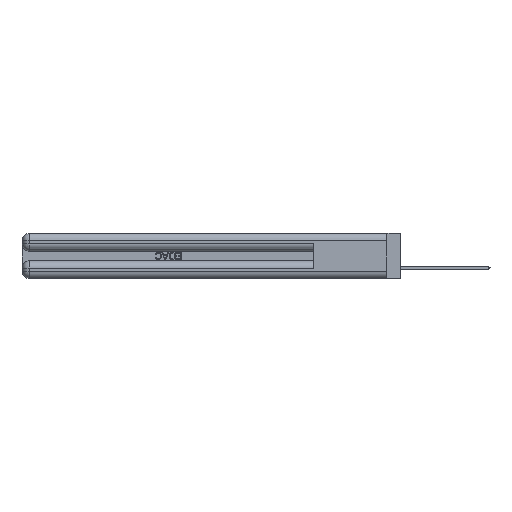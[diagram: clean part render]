
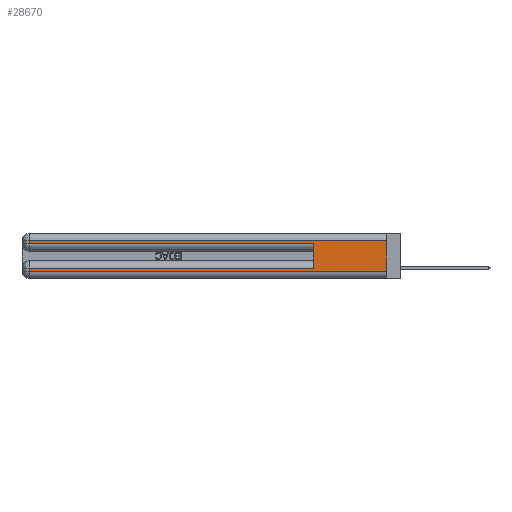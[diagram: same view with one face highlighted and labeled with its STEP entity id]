
A CAD part, left-side view. The second image highlights one B-rep face of the part: STEP entity #28670.
In plain terms, the highlighted planar face has unit normal (-1, 0, 0).
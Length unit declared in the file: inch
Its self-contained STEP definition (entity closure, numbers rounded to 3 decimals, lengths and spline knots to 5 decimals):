
#838 = LINE ( 'NONE', #39838, #31116 ) ;
#1566 = CARTESIAN_POINT ( 'NONE',  ( 0., 0., 0.06 ) ) ;
#2603 = ORIENTED_EDGE ( 'NONE', *, *, #37672, .T. ) ;
#4726 = EDGE_CURVE ( 'NONE', #37683, #33486, #39087, .T. ) ;
#4787 = DIRECTION ( 'NONE',  ( 0., 0., -1. ) ) ;
#5540 = EDGE_CURVE ( 'NONE', #25078, #27261, #838, .T. ) ;
#6211 = EDGE_CURVE ( 'NONE', #29600, #9034, #29809, .T. ) ;
#7579 = ORIENTED_EDGE ( 'NONE', *, *, #5540, .T. ) ;
#7626 = CARTESIAN_POINT ( 'NONE',  ( 0., 0., 0.31 ) ) ;
#9034 = VERTEX_POINT ( 'NONE', #51899 ) ;
#10256 = LINE ( 'NONE', #52626, #50866 ) ;
#10960 = DIRECTION ( 'NONE',  ( 0., 0., -1. ) ) ;
#11954 = VERTEX_POINT ( 'NONE', #41905 ) ;
#14354 = DIRECTION ( 'NONE',  ( 0., -1., 0. ) ) ;
#14415 = DIRECTION ( 'NONE',  ( 0., 0., -1. ) ) ;
#14491 = VERTEX_POINT ( 'NONE', #33347 ) ;
#14718 = EDGE_CURVE ( 'NONE', #33486, #11954, #10256, .T. ) ;
#15306 = VECTOR ( 'NONE', #31317, 39.37008 ) ;
#17537 = LINE ( 'NONE', #25995, #37927 ) ;
#17600 = EDGE_CURVE ( 'NONE', #25078, #14491, #49969, .T. ) ;
#18383 = DIRECTION ( 'NONE',  ( 0., 1., 0. ) ) ;
#19754 = CARTESIAN_POINT ( 'NONE',  ( 0., 0., 0.31 ) ) ;
#23510 = CARTESIAN_POINT ( 'NONE',  ( 0., 0.6, 0.145 ) ) ;
#24225 = CARTESIAN_POINT ( 'NONE',  ( 0., 2.94, 0.06 ) ) ;
#24776 = ORIENTED_EDGE ( 'NONE', *, *, #51958, .T. ) ;
#25078 = VERTEX_POINT ( 'NONE', #26284 ) ;
#25995 = CARTESIAN_POINT ( 'NONE',  ( 0., 0., 0.285 ) ) ;
#26229 = ORIENTED_EDGE ( 'NONE', *, *, #53103, .F. ) ;
#26284 = CARTESIAN_POINT ( 'NONE',  ( 0., 0.6, 0.085 ) ) ;
#27261 = VERTEX_POINT ( 'NONE', #42599 ) ;
#28142 = VECTOR ( 'NONE', #10960, 39.37008 ) ;
#28670 = ADVANCED_FACE ( 'NONE', ( #39595 ), #37199, .F. ) ;
#28828 = ORIENTED_EDGE ( 'NONE', *, *, #17600, .F. ) ;
#29336 = CARTESIAN_POINT ( 'NONE',  ( 0., 2.94, 0.37 ) ) ;
#29600 = VERTEX_POINT ( 'NONE', #24225 ) ;
#29809 = LINE ( 'NONE', #1566, #53982 ) ;
#30137 = CARTESIAN_POINT ( 'NONE',  ( 0., 0., 0.37 ) ) ;
#31116 = VECTOR ( 'NONE', #18383, 39.37008 ) ;
#31317 = DIRECTION ( 'NONE',  ( 0., 0., 1. ) ) ;
#32068 = ORIENTED_EDGE ( 'NONE', *, *, #14718, .T. ) ;
#32858 = LINE ( 'NONE', #29336, #53709 ) ;
#33347 = CARTESIAN_POINT ( 'NONE',  ( 0., 0.6, 0.285 ) ) ;
#33366 = LINE ( 'NONE', #44108, #28142 ) ;
#33486 = VERTEX_POINT ( 'NONE', #34590 ) ;
#34295 = DIRECTION ( 'NONE',  ( 0., -1., 0. ) ) ;
#34590 = CARTESIAN_POINT ( 'NONE',  ( 0., 2.94, 0.31 ) ) ;
#34769 = DIRECTION ( 'NONE',  ( 0., 1., 0. ) ) ;
#37199 = PLANE ( 'NONE',  #48744 ) ;
#37672 = EDGE_CURVE ( 'NONE', #11954, #14491, #17537, .T. ) ;
#37683 = VERTEX_POINT ( 'NONE', #7626 ) ;
#37927 = VECTOR ( 'NONE', #34295, 39.37008 ) ;
#39087 = LINE ( 'NONE', #19754, #48954 ) ;
#39595 = FACE_OUTER_BOUND ( 'NONE', #45349, .T. ) ;
#39838 = CARTESIAN_POINT ( 'NONE',  ( 0., 0., 0.085 ) ) ;
#41905 = CARTESIAN_POINT ( 'NONE',  ( 0., 2.94, 0.285 ) ) ;
#42599 = CARTESIAN_POINT ( 'NONE',  ( 0., 2.94, 0.085 ) ) ;
#43745 = ORIENTED_EDGE ( 'NONE', *, *, #6211, .T. ) ;
#44108 = CARTESIAN_POINT ( 'NONE',  ( 0., 0., 0.37 ) ) ;
#44992 = ORIENTED_EDGE ( 'NONE', *, *, #4726, .T. ) ;
#45349 = EDGE_LOOP ( 'NONE', ( #26229, #44992, #32068, #2603, #28828, #7579, #24776, #43745 ) ) ;
#48744 = AXIS2_PLACEMENT_3D ( 'NONE', #30137, #50741, #4787 ) ;
#48954 = VECTOR ( 'NONE', #34769, 39.37008 ) ;
#49969 = LINE ( 'NONE', #23510, #15306 ) ;
#50741 = DIRECTION ( 'NONE',  ( 1., 0., 0. ) ) ;
#50765 = DIRECTION ( 'NONE',  ( 0., 0., -1. ) ) ;
#50866 = VECTOR ( 'NONE', #14415, 39.37008 ) ;
#51899 = CARTESIAN_POINT ( 'NONE',  ( 0., 0., 0.06 ) ) ;
#51958 = EDGE_CURVE ( 'NONE', #27261, #29600, #32858, .T. ) ;
#52626 = CARTESIAN_POINT ( 'NONE',  ( 0., 2.94, 0.37 ) ) ;
#53103 = EDGE_CURVE ( 'NONE', #37683, #9034, #33366, .T. ) ;
#53709 = VECTOR ( 'NONE', #50765, 39.37008 ) ;
#53982 = VECTOR ( 'NONE', #14354, 39.37008 ) ;
